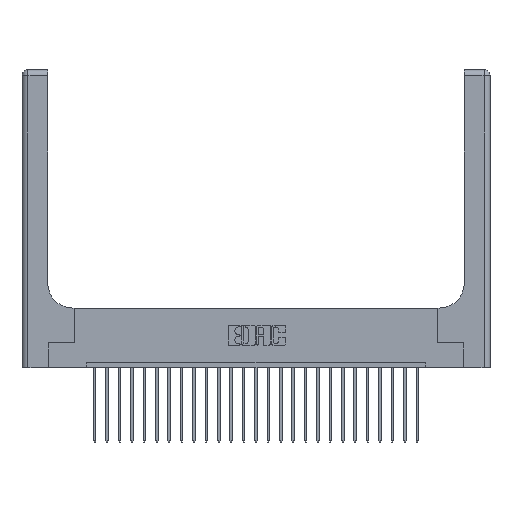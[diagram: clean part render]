
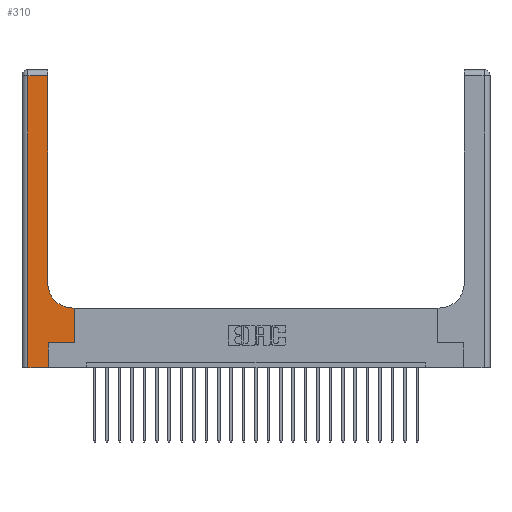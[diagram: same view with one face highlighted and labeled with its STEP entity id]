
A CAD part, top view. The second image highlights one B-rep face of the part: STEP entity #310.
In plain terms, the highlighted planar face has unit normal (0, 0, 1).
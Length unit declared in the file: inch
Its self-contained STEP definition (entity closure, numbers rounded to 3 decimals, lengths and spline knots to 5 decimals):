
#74 = VERTEX_POINT ( 'NONE', #16186 ) ;
#310 = ADVANCED_FACE ( 'NONE', ( #7306 ), #14687, .F. ) ;
#797 = ORIENTED_EDGE ( 'NONE', *, *, #13213, .T. ) ;
#1058 = AXIS2_PLACEMENT_3D ( 'NONE', #3030, #19710, #8640 ) ;
#1955 = LINE ( 'NONE', #18224, #15611 ) ;
#2244 = CARTESIAN_POINT ( 'NONE',  ( 0., 2.94, 0.37 ) ) ;
#2299 = ORIENTED_EDGE ( 'NONE', *, *, #17944, .T. ) ;
#2478 = DIRECTION ( 'NONE',  ( 0., 1., 0. ) ) ;
#2729 = DIRECTION ( 'NONE',  ( -1., 0., 0. ) ) ;
#2968 = EDGE_CURVE ( 'NONE', #4590, #74, #1955, .T. ) ;
#3030 = CARTESIAN_POINT ( 'NONE',  ( 0.51, 0.85, 0.37 ) ) ;
#3414 = EDGE_CURVE ( 'NONE', #3987, #18780, #13837, .T. ) ;
#3441 = CARTESIAN_POINT ( 'NONE',  ( 0.26, 2.94, 0.37 ) ) ;
#3512 = CARTESIAN_POINT ( 'NONE',  ( 0.06, 0., 0.37 ) ) ;
#3906 = VECTOR ( 'NONE', #8573, 39.37008 ) ;
#3987 = VERTEX_POINT ( 'NONE', #6014 ) ;
#4590 = VERTEX_POINT ( 'NONE', #21060 ) ;
#5518 = ORIENTED_EDGE ( 'NONE', *, *, #2968, .T. ) ;
#5767 = DIRECTION ( 'NONE',  ( -1., 0., 0. ) ) ;
#5797 = ORIENTED_EDGE ( 'NONE', *, *, #5857, .T. ) ;
#5857 = EDGE_CURVE ( 'NONE', #21890, #12525, #19536, .T. ) ;
#6014 = CARTESIAN_POINT ( 'NONE',  ( 0.06, 2.94, 0.37 ) ) ;
#6132 = LINE ( 'NONE', #2244, #20869 ) ;
#6335 = EDGE_CURVE ( 'NONE', #20979, #20125, #8828, .T. ) ;
#6449 = LINE ( 'NONE', #23828, #14524 ) ;
#6995 = EDGE_CURVE ( 'NONE', #20125, #4590, #7931, .T. ) ;
#7306 = FACE_OUTER_BOUND ( 'NONE', #17257, .T. ) ;
#7931 = LINE ( 'NONE', #18924, #19186 ) ;
#8573 = DIRECTION ( 'NONE',  ( 1., 0., 0. ) ) ;
#8640 = DIRECTION ( 'NONE',  ( 1., 0., 0. ) ) ;
#8828 = LINE ( 'NONE', #13909, #3906 ) ;
#9201 = CARTESIAN_POINT ( 'NONE',  ( 0., 3., 0.37 ) ) ;
#9353 = LINE ( 'NONE', #15469, #20915 ) ;
#9359 = CARTESIAN_POINT ( 'NONE',  ( 0.06, 3., 0.37 ) ) ;
#9490 = ORIENTED_EDGE ( 'NONE', *, *, #3414, .T. ) ;
#10031 = DIRECTION ( 'NONE',  ( 1., 0., 0. ) ) ;
#10174 = CARTESIAN_POINT ( 'NONE',  ( 0.265, 0.25, 0.37 ) ) ;
#12525 = VERTEX_POINT ( 'NONE', #3441 ) ;
#12912 = DIRECTION ( 'NONE',  ( 0., 0., -1. ) ) ;
#13003 = EDGE_CURVE ( 'NONE', #14739, #20979, #6449, .T. ) ;
#13213 = EDGE_CURVE ( 'NONE', #18780, #14739, #9353, .T. ) ;
#13524 = ORIENTED_EDGE ( 'NONE', *, *, #13003, .T. ) ;
#13548 = ORIENTED_EDGE ( 'NONE', *, *, #6335, .T. ) ;
#13837 = LINE ( 'NONE', #9359, #22798 ) ;
#13909 = CARTESIAN_POINT ( 'NONE',  ( 0.265, 0.25, 0.37 ) ) ;
#13940 = ORIENTED_EDGE ( 'NONE', *, *, #14328, .T. ) ;
#14328 = EDGE_CURVE ( 'NONE', #12525, #3987, #6132, .T. ) ;
#14524 = VECTOR ( 'NONE', #16626, 39.37008 ) ;
#14606 = CARTESIAN_POINT ( 'NONE',  ( 0.26, 0.85, 0.37 ) ) ;
#14687 = PLANE ( 'NONE',  #24003 ) ;
#14690 = DIRECTION ( 'NONE',  ( 0., -1., 0. ) ) ;
#14739 = VERTEX_POINT ( 'NONE', #17104 ) ;
#15469 = CARTESIAN_POINT ( 'NONE',  ( 0., 0., 0.37 ) ) ;
#15611 = VECTOR ( 'NONE', #2729, 39.37008 ) ;
#15943 = CIRCLE ( 'NONE', #1058, 0.25 ) ;
#16186 = CARTESIAN_POINT ( 'NONE',  ( 0.51, 0.6, 0.37 ) ) ;
#16388 = VECTOR ( 'NONE', #19588, 39.37008 ) ;
#16626 = DIRECTION ( 'NONE',  ( 0., 1., 0. ) ) ;
#17104 = CARTESIAN_POINT ( 'NONE',  ( 0.265, 0., 0.37 ) ) ;
#17257 = EDGE_LOOP ( 'NONE', ( #5797, #13940, #9490, #797, #13524, #13548, #22467, #5518, #2299 ) ) ;
#17520 = CARTESIAN_POINT ( 'NONE',  ( 0.26, 3., 0.37 ) ) ;
#17944 = EDGE_CURVE ( 'NONE', #74, #21890, #15943, .T. ) ;
#18224 = CARTESIAN_POINT ( 'NONE',  ( 0.26, 0.6, 0.37 ) ) ;
#18780 = VERTEX_POINT ( 'NONE', #3512 ) ;
#18924 = CARTESIAN_POINT ( 'NONE',  ( 0.528, 0.25, 0.37 ) ) ;
#19186 = VECTOR ( 'NONE', #2478, 39.37008 ) ;
#19536 = LINE ( 'NONE', #17520, #16388 ) ;
#19588 = DIRECTION ( 'NONE',  ( 0., 1., 0. ) ) ;
#19710 = DIRECTION ( 'NONE',  ( 0., 0., -1. ) ) ;
#19745 = CARTESIAN_POINT ( 'NONE',  ( 0.528, 0.25, 0.37 ) ) ;
#20125 = VERTEX_POINT ( 'NONE', #19745 ) ;
#20256 = DIRECTION ( 'NONE',  ( -1., 0., 0. ) ) ;
#20869 = VECTOR ( 'NONE', #5767, 39.37008 ) ;
#20915 = VECTOR ( 'NONE', #10031, 39.37008 ) ;
#20979 = VERTEX_POINT ( 'NONE', #10174 ) ;
#21060 = CARTESIAN_POINT ( 'NONE',  ( 0.528, 0.6, 0.37 ) ) ;
#21890 = VERTEX_POINT ( 'NONE', #14606 ) ;
#22467 = ORIENTED_EDGE ( 'NONE', *, *, #6995, .T. ) ;
#22798 = VECTOR ( 'NONE', #14690, 39.37008 ) ;
#23828 = CARTESIAN_POINT ( 'NONE',  ( 0.265, 0., 0.37 ) ) ;
#24003 = AXIS2_PLACEMENT_3D ( 'NONE', #9201, #12912, #20256 ) ;
